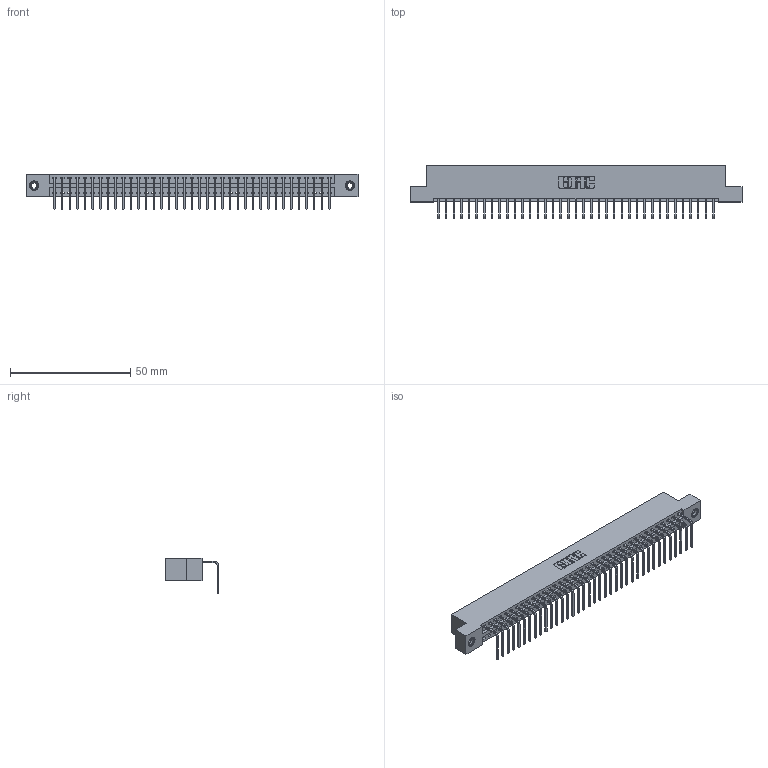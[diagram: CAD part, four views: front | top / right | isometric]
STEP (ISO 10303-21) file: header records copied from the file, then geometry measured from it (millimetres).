
FILE_DESCRIPTION (( 'STEP AP203' ), '1' );
FILE_NAME ('396-037-558-108.STEP', '2019-11-01T07:29:24', ( '' ), ( '' ), 'SwSTEP 2.0', 'SolidWorks 2016', '' );
FILE_SCHEMA (( 'CONFIG_CONTROL_DESIGN' ));
Length unit declared in the file: inch
Products named in the file (4): 345-292-001_558 Tail - 2; 345-250-001_345-250-003-102; 396-037-558-108; 346 Part_Flush Mounting Lugs - 0.156 Dia-TI
Assembly tree (40 placements, depth 2):
  396-037-558-108
    346 Part_Flush Mounting Lugs - 0.156 Dia-TI
    345-292-001_558 Tail - 2  x37
    345-250-001_345-250-003-102  x2
Bounding box: 138.05 x 22.16 x 14.73 mm (x, y, z)
Volume: 13296.7 mm3; surface area: 17322.4 mm2
Topology: 40 solids, 40 shells, 2402 faces, 7199 edges, 4742 vertices
Faces by surface type: plane 1662, cylinder 724, cone 12, torus 4
Entity records: 24906 total; most frequent: CARTESIAN_POINT 4254, ORIENTED_EDGE 4218, DIRECTION 3785, EDGE_CURVE 2109, VECTOR 1809, LINE 1809, VERTEX_POINT 1400, AXIS2_PLACEMENT_3D 988
